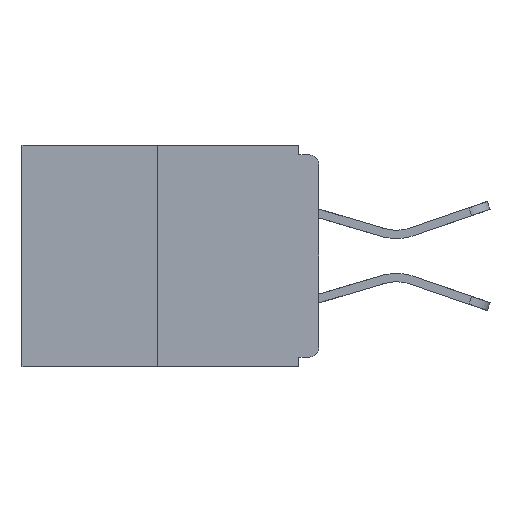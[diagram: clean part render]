
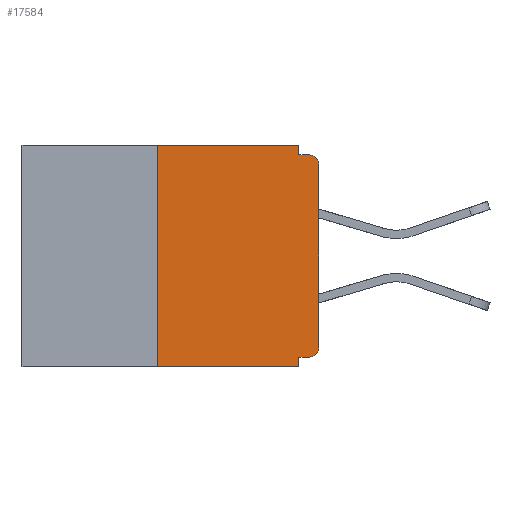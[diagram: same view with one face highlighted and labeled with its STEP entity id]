
A CAD part, left-side view. The second image highlights one B-rep face of the part: STEP entity #17584.
In plain terms, the highlighted planar face has unit normal (-1, 0, 0).
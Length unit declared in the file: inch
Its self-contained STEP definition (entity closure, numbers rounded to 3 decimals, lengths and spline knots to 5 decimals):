
#244 = DIRECTION ( 'NONE',  ( 0., 0., -1. ) ) ;
#813 = VERTEX_POINT ( 'NONE', #24802 ) ;
#1437 = VERTEX_POINT ( 'NONE', #27863 ) ;
#1591 = DIRECTION ( 'NONE',  ( 0., -1., 0. ) ) ;
#1961 = VERTEX_POINT ( 'NONE', #2615 ) ;
#2040 = CARTESIAN_POINT ( 'NONE',  ( 0., 0.031, 0. ) ) ;
#2615 = CARTESIAN_POINT ( 'NONE',  ( 0., 0.25, 0. ) ) ;
#2922 = DIRECTION ( 'NONE',  ( -1., 0., 0. ) ) ;
#3120 = CARTESIAN_POINT ( 'NONE',  ( 0., 0., -0.328 ) ) ;
#3874 = FACE_OUTER_BOUND ( 'NONE', #7869, .T. ) ;
#4252 = DIRECTION ( 'NONE',  ( 1., 0., 0. ) ) ;
#4708 = LINE ( 'NONE', #5382, #21347 ) ;
#4733 = LINE ( 'NONE', #23006, #27128 ) ;
#4824 = CARTESIAN_POINT ( 'NONE',  ( 0., 0., -0.03 ) ) ;
#4841 = AXIS2_PLACEMENT_3D ( 'NONE', #20173, #2922, #7777 ) ;
#5382 = CARTESIAN_POINT ( 'NONE',  ( 0., 0.46, 0. ) ) ;
#5394 = ORIENTED_EDGE ( 'NONE', *, *, #9059, .F. ) ;
#5874 = LINE ( 'NONE', #26230, #11960 ) ;
#6122 = DIRECTION ( 'NONE',  ( 0., 1., 0. ) ) ;
#6339 = DIRECTION ( 'NONE',  ( 0., 0., 1. ) ) ;
#7234 = LINE ( 'NONE', #2040, #18073 ) ;
#7576 = DIRECTION ( 'NONE',  ( 0., -1., 0. ) ) ;
#7777 = DIRECTION ( 'NONE',  ( 0., 0., -1. ) ) ;
#7869 = EDGE_LOOP ( 'NONE', ( #17985, #25313, #14293, #18501, #5394, #9741, #24448, #11374, #20053, #19410 ) ) ;
#9059 = EDGE_CURVE ( 'NONE', #24156, #15428, #9578, .T. ) ;
#9578 = LINE ( 'NONE', #3120, #14676 ) ;
#9741 = ORIENTED_EDGE ( 'NONE', *, *, #23927, .T. ) ;
#10230 = CARTESIAN_POINT ( 'NONE',  ( 0., 0.031, -0.343 ) ) ;
#10477 = EDGE_CURVE ( 'NONE', #1961, #24835, #4708, .T. ) ;
#10819 = DIRECTION ( 'NONE',  ( 0., 0., 1. ) ) ;
#11374 = ORIENTED_EDGE ( 'NONE', *, *, #12138, .T. ) ;
#11960 = VECTOR ( 'NONE', #244, 39.37008 ) ;
#12138 = EDGE_CURVE ( 'NONE', #20170, #1437, #26054, .T. ) ;
#12158 = CARTESIAN_POINT ( 'NONE',  ( 0., 0.031, -0.328 ) ) ;
#12417 = EDGE_CURVE ( 'NONE', #24835, #813, #7234, .T. ) ;
#12991 = CARTESIAN_POINT ( 'NONE',  ( 0., 0.25, 0. ) ) ;
#13092 = DIRECTION ( 'NONE',  ( 0., 0., -1. ) ) ;
#14096 = EDGE_CURVE ( 'NONE', #813, #1437, #4733, .T. ) ;
#14293 = ORIENTED_EDGE ( 'NONE', *, *, #26635, .T. ) ;
#14453 = DIRECTION ( 'NONE',  ( -1., 0., 0. ) ) ;
#14676 = VECTOR ( 'NONE', #6122, 39.37008 ) ;
#14847 = VECTOR ( 'NONE', #6339, 39.37008 ) ;
#14867 = LINE ( 'NONE', #25479, #22983 ) ;
#14893 = CARTESIAN_POINT ( 'NONE',  ( 0., 0., 0. ) ) ;
#15198 = PLANE ( 'NONE',  #21689 ) ;
#15377 = CARTESIAN_POINT ( 'NONE',  ( 0., 0.031, 0. ) ) ;
#15428 = VERTEX_POINT ( 'NONE', #12158 ) ;
#16160 = AXIS2_PLACEMENT_3D ( 'NONE', #21534, #14453, #27133 ) ;
#16653 = DIRECTION ( 'NONE',  ( 0., -1., 0. ) ) ;
#17180 = CARTESIAN_POINT ( 'NONE',  ( 0., 0.015, -0.328 ) ) ;
#17450 = CIRCLE ( 'NONE', #16160, 0.015 ) ;
#17584 = ADVANCED_FACE ( 'NONE', ( #3874 ), #15198, .F. ) ;
#17766 = LINE ( 'NONE', #12991, #21497 ) ;
#17985 = ORIENTED_EDGE ( 'NONE', *, *, #10477, .F. ) ;
#18073 = VECTOR ( 'NONE', #23449, 39.37008 ) ;
#18501 = ORIENTED_EDGE ( 'NONE', *, *, #19235, .F. ) ;
#18655 = VERTEX_POINT ( 'NONE', #10230 ) ;
#18715 = EDGE_CURVE ( 'NONE', #22987, #1961, #17766, .T. ) ;
#19235 = EDGE_CURVE ( 'NONE', #15428, #18655, #5874, .T. ) ;
#19410 = ORIENTED_EDGE ( 'NONE', *, *, #12417, .F. ) ;
#19451 = VERTEX_POINT ( 'NONE', #27210 ) ;
#20053 = ORIENTED_EDGE ( 'NONE', *, *, #14096, .F. ) ;
#20170 = VERTEX_POINT ( 'NONE', #4824 ) ;
#20173 = CARTESIAN_POINT ( 'NONE',  ( 0., 0.015, -0.03 ) ) ;
#20290 = LINE ( 'NONE', #14893, #14847 ) ;
#21347 = VECTOR ( 'NONE', #7576, 39.37008 ) ;
#21497 = VECTOR ( 'NONE', #10819, 39.37008 ) ;
#21534 = CARTESIAN_POINT ( 'NONE',  ( 0., 0.015, -0.313 ) ) ;
#21689 = AXIS2_PLACEMENT_3D ( 'NONE', #26289, #4252, #13092 ) ;
#22983 = VECTOR ( 'NONE', #16653, 39.37008 ) ;
#22987 = VERTEX_POINT ( 'NONE', #24190 ) ;
#23006 = CARTESIAN_POINT ( 'NONE',  ( 0., 0., -0.015 ) ) ;
#23449 = DIRECTION ( 'NONE',  ( 0., 0., -1. ) ) ;
#23927 = EDGE_CURVE ( 'NONE', #24156, #19451, #17450, .T. ) ;
#24156 = VERTEX_POINT ( 'NONE', #17180 ) ;
#24190 = CARTESIAN_POINT ( 'NONE',  ( 0., 0.25, -0.343 ) ) ;
#24448 = ORIENTED_EDGE ( 'NONE', *, *, #27440, .T. ) ;
#24802 = CARTESIAN_POINT ( 'NONE',  ( 0., 0.031, -0.015 ) ) ;
#24835 = VERTEX_POINT ( 'NONE', #15377 ) ;
#25313 = ORIENTED_EDGE ( 'NONE', *, *, #18715, .F. ) ;
#25479 = CARTESIAN_POINT ( 'NONE',  ( 0., 0.46, -0.343 ) ) ;
#26054 = CIRCLE ( 'NONE', #4841, 0.015 ) ;
#26230 = CARTESIAN_POINT ( 'NONE',  ( 0., 0.031, -0.343 ) ) ;
#26289 = CARTESIAN_POINT ( 'NONE',  ( 0., 0.46, 0. ) ) ;
#26635 = EDGE_CURVE ( 'NONE', #22987, #18655, #14867, .T. ) ;
#27128 = VECTOR ( 'NONE', #1591, 39.37008 ) ;
#27133 = DIRECTION ( 'NONE',  ( 0., 0., -1. ) ) ;
#27210 = CARTESIAN_POINT ( 'NONE',  ( 0., 0., -0.313 ) ) ;
#27440 = EDGE_CURVE ( 'NONE', #19451, #20170, #20290, .T. ) ;
#27863 = CARTESIAN_POINT ( 'NONE',  ( 0., 0.015, -0.015 ) ) ;
